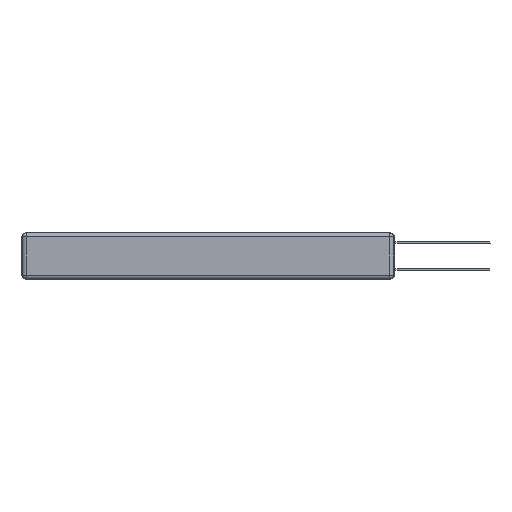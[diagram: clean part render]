
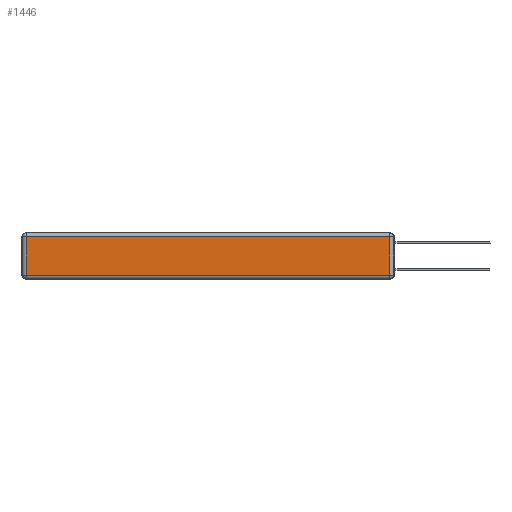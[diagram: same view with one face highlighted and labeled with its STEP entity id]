
A CAD part, left-side view. The second image highlights one B-rep face of the part: STEP entity #1446.
In plain terms, the highlighted planar face has unit normal (-1, 0, 0).
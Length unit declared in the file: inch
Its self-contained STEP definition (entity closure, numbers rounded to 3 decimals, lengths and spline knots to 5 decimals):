
#601 = VERTEX_POINT ( 'NONE', #19592 ) ;
#1038 = ORIENTED_EDGE ( 'NONE', *, *, #21749, .T. ) ;
#1230 = CARTESIAN_POINT ( 'NONE',  ( 0., 0.03, -0.343 ) ) ;
#1446 = ADVANCED_FACE ( 'NONE', ( #16420 ), #20881, .T. ) ;
#5547 = DIRECTION ( 'NONE',  ( 0., 0., 1. ) ) ;
#6052 = AXIS2_PLACEMENT_3D ( 'NONE', #14390, #7725, #14204 ) ;
#7725 = DIRECTION ( 'NONE',  ( -1., 0., 0. ) ) ;
#7864 = LINE ( 'NONE', #23324, #24721 ) ;
#8003 = LINE ( 'NONE', #25484, #12693 ) ;
#8259 = VERTEX_POINT ( 'NONE', #12051 ) ;
#8419 = CARTESIAN_POINT ( 'NONE',  ( 0., 2.72, -0.03 ) ) ;
#9411 = CARTESIAN_POINT ( 'NONE',  ( 0., 0., -0.313 ) ) ;
#11149 = VECTOR ( 'NONE', #15622, 39.37008 ) ;
#11976 = VECTOR ( 'NONE', #5547, 39.37008 ) ;
#12051 = CARTESIAN_POINT ( 'NONE',  ( 0., 0.03, -0.313 ) ) ;
#12567 = VERTEX_POINT ( 'NONE', #8419 ) ;
#12693 = VECTOR ( 'NONE', #23502, 39.37008 ) ;
#14204 = DIRECTION ( 'NONE',  ( 0., 0., 1. ) ) ;
#14254 = CARTESIAN_POINT ( 'NONE',  ( 0., 2.72, -0.313 ) ) ;
#14390 = CARTESIAN_POINT ( 'NONE',  ( 0., 0., -0.343 ) ) ;
#15622 = DIRECTION ( 'NONE',  ( 0., -1., 0. ) ) ;
#16378 = VERTEX_POINT ( 'NONE', #14254 ) ;
#16420 = FACE_OUTER_BOUND ( 'NONE', #23167, .T. ) ;
#18107 = ORIENTED_EDGE ( 'NONE', *, *, #24135, .T. ) ;
#18253 = ORIENTED_EDGE ( 'NONE', *, *, #23691, .T. ) ;
#18674 = EDGE_CURVE ( 'NONE', #12567, #16378, #7864, .T. ) ;
#19592 = CARTESIAN_POINT ( 'NONE',  ( 0., 0.03, -0.03 ) ) ;
#20881 = PLANE ( 'NONE',  #6052 ) ;
#21749 = EDGE_CURVE ( 'NONE', #16378, #8259, #26317, .T. ) ;
#22756 = LINE ( 'NONE', #1230, #11976 ) ;
#23167 = EDGE_LOOP ( 'NONE', ( #1038, #18107, #18253, #23906 ) ) ;
#23324 = CARTESIAN_POINT ( 'NONE',  ( 0., 2.72, -0.343 ) ) ;
#23502 = DIRECTION ( 'NONE',  ( 0., 1., 0. ) ) ;
#23691 = EDGE_CURVE ( 'NONE', #601, #12567, #8003, .T. ) ;
#23906 = ORIENTED_EDGE ( 'NONE', *, *, #18674, .T. ) ;
#24135 = EDGE_CURVE ( 'NONE', #8259, #601, #22756, .T. ) ;
#24721 = VECTOR ( 'NONE', #25673, 39.37008 ) ;
#25484 = CARTESIAN_POINT ( 'NONE',  ( 0., 2.75, -0.03 ) ) ;
#25673 = DIRECTION ( 'NONE',  ( 0., 0., -1. ) ) ;
#26317 = LINE ( 'NONE', #9411, #11149 ) ;
